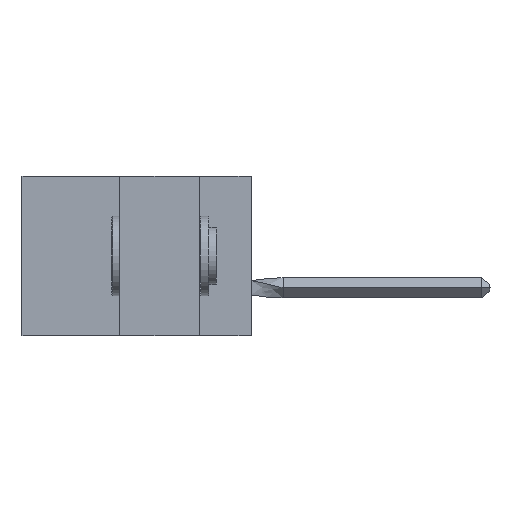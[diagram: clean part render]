
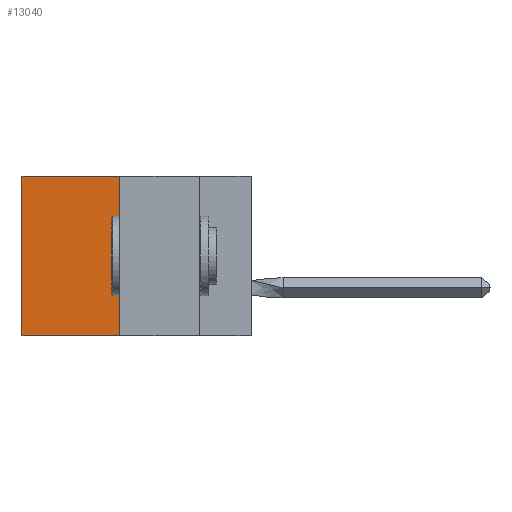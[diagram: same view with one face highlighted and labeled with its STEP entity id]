
A CAD part, left-side view. The second image highlights one B-rep face of the part: STEP entity #13040.
In plain terms, the highlighted planar face has unit normal (-1, 0, 0).
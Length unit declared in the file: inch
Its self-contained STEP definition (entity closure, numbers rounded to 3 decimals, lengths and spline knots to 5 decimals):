
#1 = CARTESIAN_POINT ( 'NONE',  ( 0.305, 0.413, -0.5 ) ) ;
#389 = VERTEX_POINT ( 'NONE', #8156 ) ;
#610 = VECTOR ( 'NONE', #17926, 39.37008 ) ;
#1264 = VECTOR ( 'NONE', #10724, 39.37008 ) ;
#2186 = CARTESIAN_POINT ( 'NONE',  ( 0.305, 0.72, -0.5 ) ) ;
#2781 = DIRECTION ( 'NONE',  ( 0., 1., 0. ) ) ;
#2863 = PLANE ( 'NONE',  #12619 ) ;
#2923 = DIRECTION ( 'NONE',  ( 0., 0., -1. ) ) ;
#3580 = ORIENTED_EDGE ( 'NONE', *, *, #15318, .F. ) ;
#4962 = LINE ( 'NONE', #15631, #14503 ) ;
#6297 = VECTOR ( 'NONE', #13562, 39.37008 ) ;
#7237 = DIRECTION ( 'NONE',  ( 1., 0., 0. ) ) ;
#7672 = EDGE_LOOP ( 'NONE', ( #12489, #3580, #17290, #10573 ) ) ;
#7702 = VERTEX_POINT ( 'NONE', #10201 ) ;
#8081 = LINE ( 'NONE', #9457, #6297 ) ;
#8156 = CARTESIAN_POINT ( 'NONE',  ( 0.305, 0.72, -0.5 ) ) ;
#8323 = LINE ( 'NONE', #17864, #610 ) ;
#9457 = CARTESIAN_POINT ( 'NONE',  ( 0.305, 0.413, -0.5 ) ) ;
#9683 = CARTESIAN_POINT ( 'NONE',  ( 0.305, 0.72, 0. ) ) ;
#9972 = CARTESIAN_POINT ( 'NONE',  ( 0.305, 0.413, 0. ) ) ;
#10201 = CARTESIAN_POINT ( 'NONE',  ( 0.305, 0.413, -0.5 ) ) ;
#10573 = ORIENTED_EDGE ( 'NONE', *, *, #14597, .T. ) ;
#10724 = DIRECTION ( 'NONE',  ( 0., 0., -1. ) ) ;
#12489 = ORIENTED_EDGE ( 'NONE', *, *, #14373, .T. ) ;
#12619 = AXIS2_PLACEMENT_3D ( 'NONE', #1, #7237, #2923 ) ;
#12783 = LINE ( 'NONE', #2186, #1264 ) ;
#13029 = VERTEX_POINT ( 'NONE', #9972 ) ;
#13040 = ADVANCED_FACE ( 'NONE', ( #16762 ), #2863, .F. ) ;
#13562 = DIRECTION ( 'NONE',  ( 0., 0., -1. ) ) ;
#14373 = EDGE_CURVE ( 'NONE', #18164, #389, #12783, .T. ) ;
#14503 = VECTOR ( 'NONE', #2781, 39.37008 ) ;
#14597 = EDGE_CURVE ( 'NONE', #13029, #18164, #8323, .T. ) ;
#15023 = EDGE_CURVE ( 'NONE', #13029, #7702, #8081, .T. ) ;
#15318 = EDGE_CURVE ( 'NONE', #7702, #389, #4962, .T. ) ;
#15631 = CARTESIAN_POINT ( 'NONE',  ( 0.305, 0.413, -0.5 ) ) ;
#16762 = FACE_OUTER_BOUND ( 'NONE', #7672, .T. ) ;
#17290 = ORIENTED_EDGE ( 'NONE', *, *, #15023, .F. ) ;
#17864 = CARTESIAN_POINT ( 'NONE',  ( 0.305, 0.413, 0. ) ) ;
#17926 = DIRECTION ( 'NONE',  ( 0., 1., 0. ) ) ;
#18164 = VERTEX_POINT ( 'NONE', #9683 ) ;
